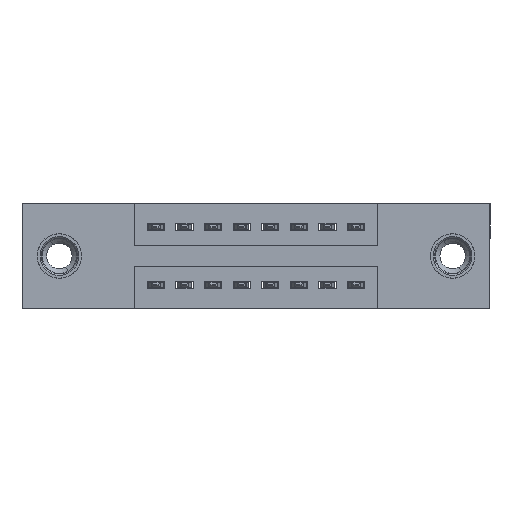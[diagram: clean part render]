
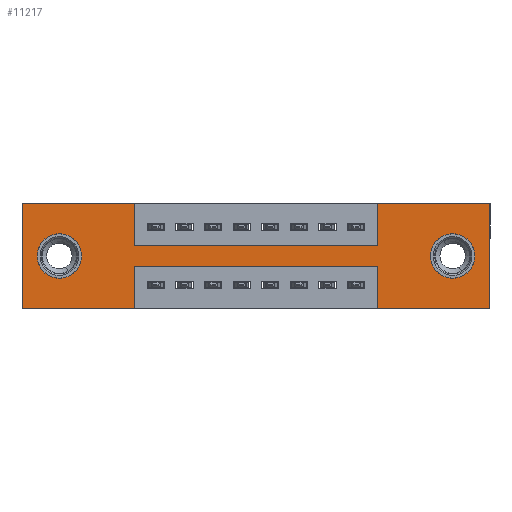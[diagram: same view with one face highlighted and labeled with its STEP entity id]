
A CAD part, front view. The second image highlights one B-rep face of the part: STEP entity #11217.
In plain terms, the highlighted planar face has unit normal (0, -1, 0).
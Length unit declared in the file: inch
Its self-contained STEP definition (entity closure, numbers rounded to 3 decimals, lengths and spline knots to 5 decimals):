
#21 = DIRECTION ( 'NONE',  ( 0., -1., 0. ) ) ;
#29 = EDGE_LOOP ( 'NONE', ( #1987, #10397 ) ) ;
#39 = DIRECTION ( 'NONE',  ( 0., 0., -1. ) ) ;
#148 = LINE ( 'NONE', #2457, #5856 ) ;
#266 = ORIENTED_EDGE ( 'NONE', *, *, #8409, .F. ) ;
#274 = CARTESIAN_POINT ( 'NONE',  ( 0.3925, 0., -0.15 ) ) ;
#280 = ORIENTED_EDGE ( 'NONE', *, *, #7130, .F. ) ;
#450 = CARTESIAN_POINT ( 'NONE',  ( 0.3925, 0., -0.22 ) ) ;
#474 = CARTESIAN_POINT ( 'NONE',  ( 1.505, 0., -0.107 ) ) ;
#539 = ORIENTED_EDGE ( 'NONE', *, *, #9176, .F. ) ;
#647 = CARTESIAN_POINT ( 'NONE',  ( 0.3925, 0., -0.37 ) ) ;
#683 = FACE_BOUND ( 'NONE', #29, .T. ) ;
#760 = VECTOR ( 'NONE', #11815, 39.37008 ) ;
#852 = AXIS2_PLACEMENT_3D ( 'NONE', #11156, #14793, #3857 ) ;
#885 = LINE ( 'NONE', #2447, #6016 ) ;
#1268 = CARTESIAN_POINT ( 'NONE',  ( 0., 0., -0.37 ) ) ;
#1475 = AXIS2_PLACEMENT_3D ( 'NONE', #7181, #2522, #7282 ) ;
#1497 = CARTESIAN_POINT ( 'NONE',  ( 0., 0., 0. ) ) ;
#1548 = EDGE_CURVE ( 'NONE', #12260, #5452, #148, .T. ) ;
#1785 = VECTOR ( 'NONE', #12215, 39.37008 ) ;
#1803 = LINE ( 'NONE', #647, #9412 ) ;
#1859 = CARTESIAN_POINT ( 'NONE',  ( 0.3925, 0., -0.37 ) ) ;
#1987 = ORIENTED_EDGE ( 'NONE', *, *, #8192, .T. ) ;
#2011 = DIRECTION ( 'NONE',  ( 0., 0., 1. ) ) ;
#2046 = AXIS2_PLACEMENT_3D ( 'NONE', #13365, #21, #8541 ) ;
#2128 = DIRECTION ( 'NONE',  ( 0., 0., -1. ) ) ;
#2447 = CARTESIAN_POINT ( 'NONE',  ( 0.3925, 0., -0.15 ) ) ;
#2457 = CARTESIAN_POINT ( 'NONE',  ( 1.635, 0., 0. ) ) ;
#2522 = DIRECTION ( 'NONE',  ( 0., 1., 0. ) ) ;
#2588 = LINE ( 'NONE', #7083, #8671 ) ;
#2614 = LINE ( 'NONE', #11180, #12700 ) ;
#2815 = ORIENTED_EDGE ( 'NONE', *, *, #12044, .F. ) ;
#2880 = CIRCLE ( 'NONE', #8175, 0.078 ) ;
#2934 = VERTEX_POINT ( 'NONE', #450 ) ;
#2995 = ORIENTED_EDGE ( 'NONE', *, *, #13344, .F. ) ;
#3313 = CARTESIAN_POINT ( 'NONE',  ( 1.2425, 0., -0.37 ) ) ;
#3857 = DIRECTION ( 'NONE',  ( 0., 0., 1. ) ) ;
#4196 = LINE ( 'NONE', #3313, #760 ) ;
#4547 = DIRECTION ( 'NONE',  ( 1., 0., 0. ) ) ;
#4640 = ORIENTED_EDGE ( 'NONE', *, *, #1548, .F. ) ;
#4869 = EDGE_CURVE ( 'NONE', #10714, #10629, #2880, .T. ) ;
#4974 = VERTEX_POINT ( 'NONE', #5768 ) ;
#5452 = VERTEX_POINT ( 'NONE', #14403 ) ;
#5712 = DIRECTION ( 'NONE',  ( 0., 1., 0. ) ) ;
#5768 = CARTESIAN_POINT ( 'NONE',  ( 0., 0., 0. ) ) ;
#5778 = ORIENTED_EDGE ( 'NONE', *, *, #15680, .F. ) ;
#5843 = LINE ( 'NONE', #1497, #12123 ) ;
#5856 = VECTOR ( 'NONE', #39, 39.37008 ) ;
#5995 = ORIENTED_EDGE ( 'NONE', *, *, #10000, .F. ) ;
#6002 = EDGE_CURVE ( 'NONE', #9197, #6804, #11212, .T. ) ;
#6016 = VECTOR ( 'NONE', #15751, 39.37008 ) ;
#6206 = ORIENTED_EDGE ( 'NONE', *, *, #6002, .F. ) ;
#6240 = AXIS2_PLACEMENT_3D ( 'NONE', #11778, #5712, #2011 ) ;
#6384 = ORIENTED_EDGE ( 'NONE', *, *, #6632, .T. ) ;
#6632 = EDGE_CURVE ( 'NONE', #10629, #10714, #10056, .T. ) ;
#6701 = LINE ( 'NONE', #11144, #13433 ) ;
#6749 = FACE_OUTER_BOUND ( 'NONE', #14109, .T. ) ;
#6804 = VERTEX_POINT ( 'NONE', #274 ) ;
#6890 = CARTESIAN_POINT ( 'NONE',  ( 1.2425, 0., -0.37 ) ) ;
#7083 = CARTESIAN_POINT ( 'NONE',  ( 0., 0., 0. ) ) ;
#7130 = EDGE_CURVE ( 'NONE', #13036, #12043, #2614, .T. ) ;
#7181 = CARTESIAN_POINT ( 'NONE',  ( 1.505, 0., -0.185 ) ) ;
#7282 = DIRECTION ( 'NONE',  ( 0., 0., -1. ) ) ;
#7529 = CARTESIAN_POINT ( 'NONE',  ( 0., 0., -0.37 ) ) ;
#7712 = EDGE_CURVE ( 'NONE', #6804, #13036, #885, .T. ) ;
#8162 = ORIENTED_EDGE ( 'NONE', *, *, #14511, .F. ) ;
#8175 = AXIS2_PLACEMENT_3D ( 'NONE', #9231, #12905, #15322 ) ;
#8192 = EDGE_CURVE ( 'NONE', #10790, #10934, #13404, .T. ) ;
#8302 = LINE ( 'NONE', #9501, #13234 ) ;
#8328 = CARTESIAN_POINT ( 'NONE',  ( 1.2425, 0., -0.22 ) ) ;
#8373 = CARTESIAN_POINT ( 'NONE',  ( 1.2425, 0., 0. ) ) ;
#8409 = EDGE_CURVE ( 'NONE', #12611, #12360, #6701, .T. ) ;
#8541 = DIRECTION ( 'NONE',  ( 0., 0., -1. ) ) ;
#8671 = VECTOR ( 'NONE', #10625, 39.37008 ) ;
#8705 = PLANE ( 'NONE',  #2046 ) ;
#8872 = CARTESIAN_POINT ( 'NONE',  ( 1.505, 0., -0.263 ) ) ;
#9033 = ORIENTED_EDGE ( 'NONE', *, *, #7712, .F. ) ;
#9176 = EDGE_CURVE ( 'NONE', #12360, #4974, #5843, .T. ) ;
#9197 = VERTEX_POINT ( 'NONE', #11230 ) ;
#9231 = CARTESIAN_POINT ( 'NONE',  ( 1.505, 0., -0.185 ) ) ;
#9321 = CIRCLE ( 'NONE', #852, 0.078 ) ;
#9350 = CARTESIAN_POINT ( 'NONE',  ( 0.3925, 0., 0. ) ) ;
#9412 = VECTOR ( 'NONE', #14087, 39.37008 ) ;
#9501 = CARTESIAN_POINT ( 'NONE',  ( 0., 0., 0. ) ) ;
#10000 = EDGE_CURVE ( 'NONE', #12043, #12260, #2588, .T. ) ;
#10056 = CIRCLE ( 'NONE', #1475, 0.078 ) ;
#10162 = CARTESIAN_POINT ( 'NONE',  ( 1.2425, 0., -0.15 ) ) ;
#10216 = DIRECTION ( 'NONE',  ( 0., 0., 1. ) ) ;
#10397 = ORIENTED_EDGE ( 'NONE', *, *, #15510, .T. ) ;
#10625 = DIRECTION ( 'NONE',  ( 1., 0., 0. ) ) ;
#10629 = VERTEX_POINT ( 'NONE', #8872 ) ;
#10714 = VERTEX_POINT ( 'NONE', #474 ) ;
#10790 = VERTEX_POINT ( 'NONE', #12757 ) ;
#10934 = VERTEX_POINT ( 'NONE', #13026 ) ;
#11018 = CARTESIAN_POINT ( 'NONE',  ( 0.3925, 0., -0.22 ) ) ;
#11144 = CARTESIAN_POINT ( 'NONE',  ( 0., 0., -0.37 ) ) ;
#11156 = CARTESIAN_POINT ( 'NONE',  ( 0.13, 0., -0.185 ) ) ;
#11180 = CARTESIAN_POINT ( 'NONE',  ( 1.2425, 0., 0. ) ) ;
#11212 = LINE ( 'NONE', #9350, #13667 ) ;
#11217 = ADVANCED_FACE ( 'NONE', ( #12666, #683, #6749 ), #8705, .T. ) ;
#11230 = CARTESIAN_POINT ( 'NONE',  ( 0.3925, 0., 0. ) ) ;
#11357 = DIRECTION ( 'NONE',  ( -1., 0., 0. ) ) ;
#11778 = CARTESIAN_POINT ( 'NONE',  ( 0.13, 0., -0.185 ) ) ;
#11815 = DIRECTION ( 'NONE',  ( 0., 0., 1. ) ) ;
#12043 = VERTEX_POINT ( 'NONE', #8373 ) ;
#12044 = EDGE_CURVE ( 'NONE', #2934, #12611, #1803, .T. ) ;
#12090 = EDGE_LOOP ( 'NONE', ( #12350, #6384 ) ) ;
#12123 = VECTOR ( 'NONE', #10216, 39.37008 ) ;
#12215 = DIRECTION ( 'NONE',  ( -1., 0., 0. ) ) ;
#12233 = EDGE_CURVE ( 'NONE', #15702, #2934, #15275, .T. ) ;
#12260 = VERTEX_POINT ( 'NONE', #13431 ) ;
#12322 = DIRECTION ( 'NONE',  ( 0., 0., 1. ) ) ;
#12350 = ORIENTED_EDGE ( 'NONE', *, *, #4869, .T. ) ;
#12360 = VERTEX_POINT ( 'NONE', #7529 ) ;
#12611 = VERTEX_POINT ( 'NONE', #1859 ) ;
#12666 = FACE_BOUND ( 'NONE', #12090, .T. ) ;
#12700 = VECTOR ( 'NONE', #12322, 39.37008 ) ;
#12757 = CARTESIAN_POINT ( 'NONE',  ( 0.13, 0., -0.107 ) ) ;
#12905 = DIRECTION ( 'NONE',  ( 0., 1., 0. ) ) ;
#13026 = CARTESIAN_POINT ( 'NONE',  ( 0.13, 0., -0.263 ) ) ;
#13036 = VERTEX_POINT ( 'NONE', #10162 ) ;
#13234 = VECTOR ( 'NONE', #4547, 39.37008 ) ;
#13316 = DIRECTION ( 'NONE',  ( -1., 0., 0. ) ) ;
#13344 = EDGE_CURVE ( 'NONE', #5452, #15108, #15433, .T. ) ;
#13365 = CARTESIAN_POINT ( 'NONE',  ( 0., 0., -0.37 ) ) ;
#13404 = CIRCLE ( 'NONE', #6240, 0.078 ) ;
#13431 = CARTESIAN_POINT ( 'NONE',  ( 1.635, 0., 0. ) ) ;
#13433 = VECTOR ( 'NONE', #11357, 39.37008 ) ;
#13667 = VECTOR ( 'NONE', #2128, 39.37008 ) ;
#13731 = ORIENTED_EDGE ( 'NONE', *, *, #12233, .F. ) ;
#14087 = DIRECTION ( 'NONE',  ( 0., 0., -1. ) ) ;
#14109 = EDGE_LOOP ( 'NONE', ( #2815, #13731, #8162, #2995, #4640, #5995, #280, #9033, #6206, #5778, #539, #266 ) ) ;
#14403 = CARTESIAN_POINT ( 'NONE',  ( 1.635, 0., -0.37 ) ) ;
#14511 = EDGE_CURVE ( 'NONE', #15108, #15702, #4196, .T. ) ;
#14793 = DIRECTION ( 'NONE',  ( 0., 1., 0. ) ) ;
#14847 = VECTOR ( 'NONE', #13316, 39.37008 ) ;
#15108 = VERTEX_POINT ( 'NONE', #6890 ) ;
#15275 = LINE ( 'NONE', #11018, #1785 ) ;
#15322 = DIRECTION ( 'NONE',  ( 0., 0., -1. ) ) ;
#15433 = LINE ( 'NONE', #1268, #14847 ) ;
#15510 = EDGE_CURVE ( 'NONE', #10934, #10790, #9321, .T. ) ;
#15680 = EDGE_CURVE ( 'NONE', #4974, #9197, #8302, .T. ) ;
#15702 = VERTEX_POINT ( 'NONE', #8328 ) ;
#15751 = DIRECTION ( 'NONE',  ( 1., 0., 0. ) ) ;
